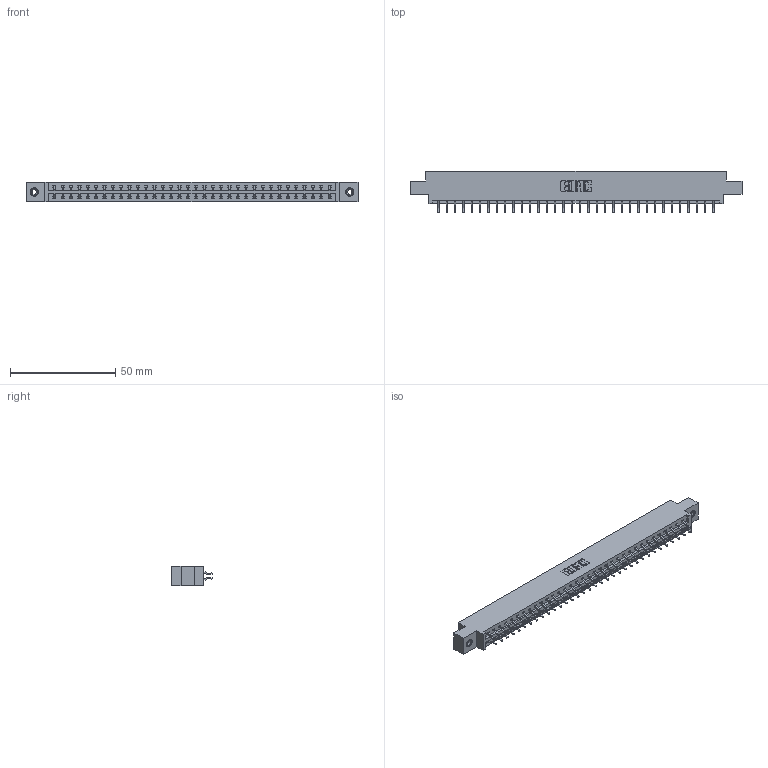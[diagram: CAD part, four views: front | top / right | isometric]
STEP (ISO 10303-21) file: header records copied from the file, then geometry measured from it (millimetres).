
FILE_DESCRIPTION (( 'STEP AP203' ), '1' );
FILE_NAME ('387-068-556-808.STEP', '2018-09-22T15:57:15', ( '' ), ( '' ), 'SwSTEP 2.0', 'SolidWorks 2016', '' );
FILE_SCHEMA (( 'CONFIG_CONTROL_DESIGN' ));
Length unit declared in the file: inch
Products named in the file (4): 387-068-556-808; 337 Part_0.170 Offset - 0.156 Dia-TI; 345-292-001_556 Tail; 345-250-001_345-250-003-102
Assembly tree (71 placements, depth 2):
  387-068-556-808
    337 Part_0.170 Offset - 0.156 Dia-TI
    345-292-001_556 Tail  x68
    345-250-001_345-250-003-102  x2
Bounding box: 157.73 x 19.57 x 9.4 mm (x, y, z)
Volume: 16390.1 mm3; surface area: 18511.3 mm2
Topology: 71 solids, 71 shells, 4258 faces, 12631 edges, 8322 vertices
Faces by surface type: plane 2962, cylinder 1280, cone 12, torus 4
Entity records: 28934 total; most frequent: CARTESIAN_POINT 4877, ORIENTED_EDGE 4794, DIRECTION 4183, EDGE_CURVE 2397, LINE 2241, VECTOR 2241, VERTEX_POINT 1592, AXIS2_PLACEMENT_3D 971
